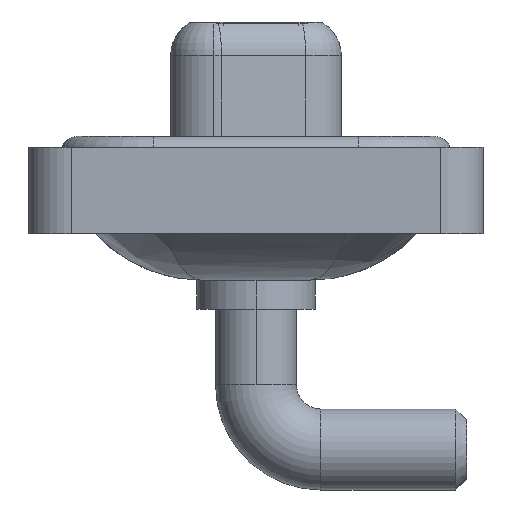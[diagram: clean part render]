
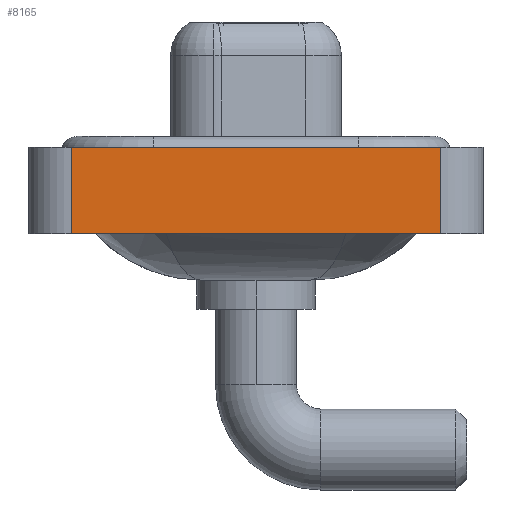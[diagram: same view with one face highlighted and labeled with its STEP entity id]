
A CAD part, left-side view. The second image highlights one B-rep face of the part: STEP entity #8165.
In plain terms, the highlighted planar face has unit normal (-1, 0, 0).
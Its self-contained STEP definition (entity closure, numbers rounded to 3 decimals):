
#221 = PLANE ( 'NONE',  #11754 ) ;
#1017 = VECTOR ( 'NONE', #1759, 1000. ) ;
#1396 = CARTESIAN_POINT ( 'NONE',  ( -7.25, -8.55, -3.6 ) ) ;
#1759 = DIRECTION ( 'NONE',  ( 0., 0., 1. ) ) ;
#1835 = CARTESIAN_POINT ( 'NONE',  ( -7.25, 8.55, 0.4 ) ) ;
#3344 = ORIENTED_EDGE ( 'NONE', *, *, #11568, .F. ) ;
#3827 = ORIENTED_EDGE ( 'NONE', *, *, #8580, .F. ) ;
#5052 = CARTESIAN_POINT ( 'NONE',  ( -7.25, -8.55, -3.6 ) ) ;
#5059 = DIRECTION ( 'NONE',  ( 0., -1., 0. ) ) ;
#5216 = DIRECTION ( 'NONE',  ( -1., 0., 0. ) ) ;
#5410 = ORIENTED_EDGE ( 'NONE', *, *, #14379, .T. ) ;
#6189 = VERTEX_POINT ( 'NONE', #11805 ) ;
#6538 = CARTESIAN_POINT ( 'NONE',  ( -7.25, -8.55, 0.4 ) ) ;
#6907 = CARTESIAN_POINT ( 'NONE',  ( -7.25, -8.55, -3.6 ) ) ;
#7379 = VERTEX_POINT ( 'NONE', #6907 ) ;
#8127 = CARTESIAN_POINT ( 'NONE',  ( -7.25, -8.55, 0.4 ) ) ;
#8165 = ADVANCED_FACE ( 'NONE', ( #8619 ), #221, .T. ) ;
#8580 = EDGE_CURVE ( 'NONE', #6189, #12264, #14593, .T. ) ;
#8619 = FACE_OUTER_BOUND ( 'NONE', #12560, .T. ) ;
#8808 = ORIENTED_EDGE ( 'NONE', *, *, #12212, .T. ) ;
#10074 = DIRECTION ( 'NONE',  ( 0., 0., 1. ) ) ;
#10722 = CARTESIAN_POINT ( 'NONE',  ( -7.25, 8.55, -3.6 ) ) ;
#11006 = VECTOR ( 'NONE', #5059, 1000. ) ;
#11355 = LINE ( 'NONE', #11427, #1017 ) ;
#11427 = CARTESIAN_POINT ( 'NONE',  ( -7.25, -8.55, -3.6 ) ) ;
#11568 = EDGE_CURVE ( 'NONE', #12264, #15540, #12002, .T. ) ;
#11754 = AXIS2_PLACEMENT_3D ( 'NONE', #5052, #5216, #10074 ) ;
#11764 = VECTOR ( 'NONE', #11895, 1000. ) ;
#11805 = CARTESIAN_POINT ( 'NONE',  ( -7.25, 8.55, -3.6 ) ) ;
#11895 = DIRECTION ( 'NONE',  ( 0., 0., 1. ) ) ;
#12002 = LINE ( 'NONE', #8127, #12767 ) ;
#12212 = EDGE_CURVE ( 'NONE', #7379, #15540, #11355, .T. ) ;
#12264 = VERTEX_POINT ( 'NONE', #1835 ) ;
#12560 = EDGE_LOOP ( 'NONE', ( #8808, #3344, #3827, #5410 ) ) ;
#12767 = VECTOR ( 'NONE', #14465, 1000. ) ;
#13386 = LINE ( 'NONE', #1396, #11006 ) ;
#14379 = EDGE_CURVE ( 'NONE', #6189, #7379, #13386, .T. ) ;
#14465 = DIRECTION ( 'NONE',  ( 0., -1., 0. ) ) ;
#14593 = LINE ( 'NONE', #10722, #11764 ) ;
#15540 = VERTEX_POINT ( 'NONE', #6538 ) ;
